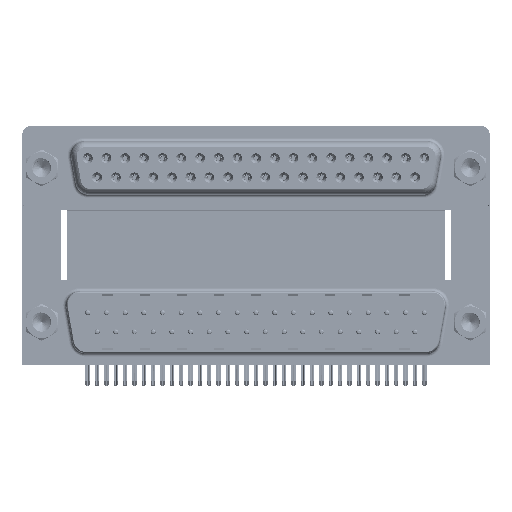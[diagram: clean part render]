
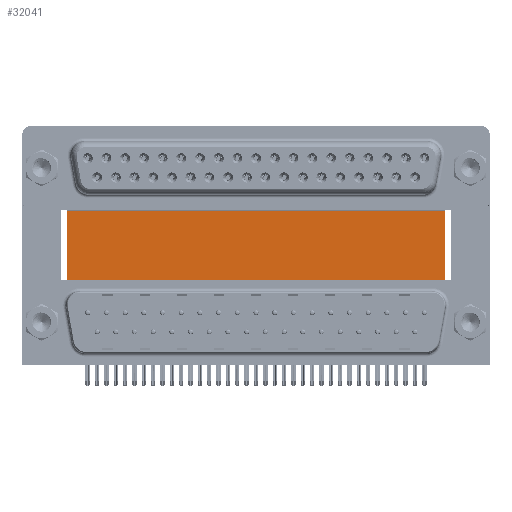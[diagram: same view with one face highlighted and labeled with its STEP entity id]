
A CAD part, top view. The second image highlights one B-rep face of the part: STEP entity #32041.
In plain terms, the highlighted planar face has unit normal (0, 0, 1).
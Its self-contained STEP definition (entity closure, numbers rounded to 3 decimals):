
#1604 = AXIS2_PLACEMENT_3D ( 'NONE', #67349, #61634, #67714 ) ;
#2611 = LINE ( 'NONE', #32559, #23940 ) ;
#6072 = VECTOR ( 'NONE', #51737, 1000. ) ;
#8189 = CARTESIAN_POINT ( 'NONE',  ( 3.79, -3.735, -12. ) ) ;
#9052 = VERTEX_POINT ( 'NONE', #72816 ) ;
#9553 = CARTESIAN_POINT ( 'NONE',  ( 59.71, 16.585, -12. ) ) ;
#9636 = CARTESIAN_POINT ( 'NONE',  ( 3.79, 16.585, -12. ) ) ;
#9689 = FACE_OUTER_BOUND ( 'NONE', #42452, .T. ) ;
#11496 = EDGE_CURVE ( 'NONE', #46520, #9052, #32936, .T. ) ;
#13185 = ORIENTED_EDGE ( 'NONE', *, *, #26635, .T. ) ;
#14776 = CARTESIAN_POINT ( 'NONE',  ( 3.79, -3.735, -12. ) ) ;
#21061 = PLANE ( 'NONE',  #1604 ) ;
#23940 = VECTOR ( 'NONE', #61354, 1000. ) ;
#26374 = DIRECTION ( 'NONE',  ( 1., 0., 0. ) ) ;
#26635 = EDGE_CURVE ( 'NONE', #72142, #34411, #58134, .T. ) ;
#32041 = ADVANCED_FACE ( 'NONE', ( #9689 ), #21061, .F. ) ;
#32559 = CARTESIAN_POINT ( 'NONE',  ( 3.79, 16.585, -12. ) ) ;
#32936 = LINE ( 'NONE', #37898, #68706 ) ;
#34411 = VERTEX_POINT ( 'NONE', #14776 ) ;
#36162 = CARTESIAN_POINT ( 'NONE',  ( 3.79, 16.585, -12. ) ) ;
#37898 = CARTESIAN_POINT ( 'NONE',  ( 59.71, 16.585, -12. ) ) ;
#42452 = EDGE_LOOP ( 'NONE', ( #72839, #46602, #53983, #13185 ) ) ;
#46520 = VERTEX_POINT ( 'NONE', #9553 ) ;
#46602 = ORIENTED_EDGE ( 'NONE', *, *, #11496, .F. ) ;
#48289 = VECTOR ( 'NONE', #26374, 1000. ) ;
#51737 = DIRECTION ( 'NONE',  ( 0., -1., 0. ) ) ;
#53983 = ORIENTED_EDGE ( 'NONE', *, *, #69767, .F. ) ;
#56318 = EDGE_CURVE ( 'NONE', #34411, #9052, #65442, .T. ) ;
#58134 = LINE ( 'NONE', #36162, #6072 ) ;
#61354 = DIRECTION ( 'NONE',  ( 1., 0., 0. ) ) ;
#61634 = DIRECTION ( 'NONE',  ( 0., 0., -1. ) ) ;
#65442 = LINE ( 'NONE', #8189, #48289 ) ;
#67349 = CARTESIAN_POINT ( 'NONE',  ( 3.79, 16.585, -12. ) ) ;
#67714 = DIRECTION ( 'NONE',  ( -1., 0., 0. ) ) ;
#68706 = VECTOR ( 'NONE', #72443, 1000. ) ;
#69767 = EDGE_CURVE ( 'NONE', #72142, #46520, #2611, .T. ) ;
#72142 = VERTEX_POINT ( 'NONE', #9636 ) ;
#72443 = DIRECTION ( 'NONE',  ( 0., -1., 0. ) ) ;
#72816 = CARTESIAN_POINT ( 'NONE',  ( 59.71, -3.735, -12. ) ) ;
#72839 = ORIENTED_EDGE ( 'NONE', *, *, #56318, .T. ) ;
